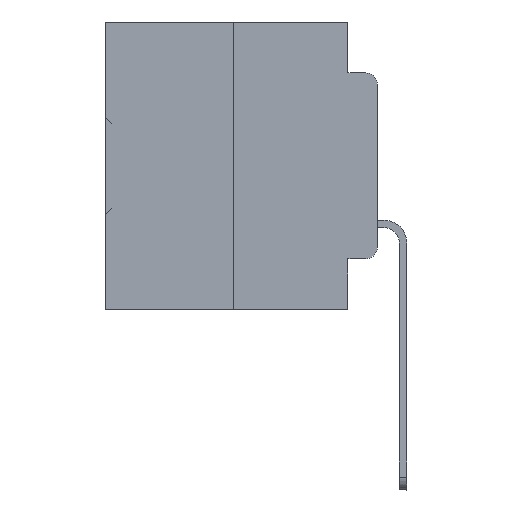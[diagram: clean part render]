
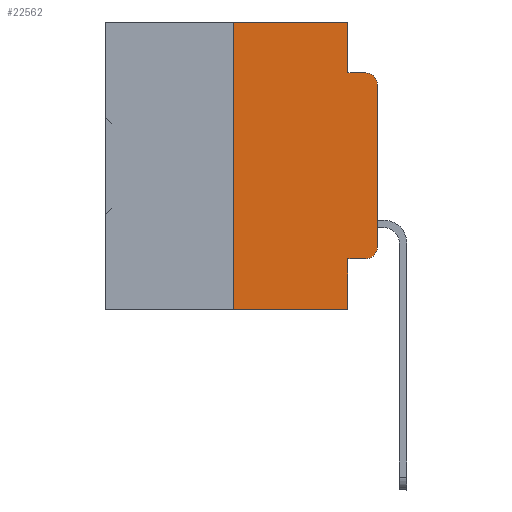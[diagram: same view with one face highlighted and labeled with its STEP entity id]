
A CAD part, left-side view. The second image highlights one B-rep face of the part: STEP entity #22562.
In plain terms, the highlighted planar face has unit normal (-1, 0, 0).
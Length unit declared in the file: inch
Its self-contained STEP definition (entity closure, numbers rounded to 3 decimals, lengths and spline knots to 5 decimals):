
#402 = CARTESIAN_POINT ( 'NONE',  ( 0., 0.473, 0. ) ) ;
#460 = EDGE_CURVE ( 'NONE', #38475, #35663, #22220, .T. ) ;
#1138 = LINE ( 'NONE', #13096, #17707 ) ;
#1702 = DIRECTION ( 'NONE',  ( 0., 0., 1. ) ) ;
#1963 = ORIENTED_EDGE ( 'NONE', *, *, #19429, .T. ) ;
#1972 = VERTEX_POINT ( 'NONE', #7918 ) ;
#2332 = CARTESIAN_POINT ( 'NONE',  ( 0., 0.02, -0.4115 ) ) ;
#2623 = AXIS2_PLACEMENT_3D ( 'NONE', #5279, #17221, #29190 ) ;
#2674 = EDGE_CURVE ( 'NONE', #1972, #4587, #21550, .T. ) ;
#2733 = CARTESIAN_POINT ( 'NONE',  ( 0., 0.051, 0. ) ) ;
#2928 = CARTESIAN_POINT ( 'NONE',  ( 0., 0.25, -0.5 ) ) ;
#3065 = VERTEX_POINT ( 'NONE', #2332 ) ;
#4380 = CARTESIAN_POINT ( 'NONE',  ( 0., 0.02, -0.1085 ) ) ;
#4405 = CARTESIAN_POINT ( 'NONE',  ( 0., 0.051, -0.0885 ) ) ;
#4587 = VERTEX_POINT ( 'NONE', #2733 ) ;
#5279 = CARTESIAN_POINT ( 'NONE',  ( 0., 0.473, 0. ) ) ;
#5509 = VECTOR ( 'NONE', #1702, 39.37008 ) ;
#7273 = DIRECTION ( 'NONE',  ( 0., 0., 1. ) ) ;
#7759 = CARTESIAN_POINT ( 'NONE',  ( 0., 0.051, 0. ) ) ;
#7784 = EDGE_CURVE ( 'NONE', #4587, #38475, #34631, .T. ) ;
#7918 = CARTESIAN_POINT ( 'NONE',  ( 0., 0.25, 0. ) ) ;
#9548 = ORIENTED_EDGE ( 'NONE', *, *, #28734, .T. ) ;
#11099 = CARTESIAN_POINT ( 'NONE',  ( 0., 0., -0.3915 ) ) ;
#11233 = ORIENTED_EDGE ( 'NONE', *, *, #2674, .F. ) ;
#11368 = FACE_OUTER_BOUND ( 'NONE', #25477, .T. ) ;
#11465 = CARTESIAN_POINT ( 'NONE',  ( 0., 0.02, -0.3915 ) ) ;
#11811 = VECTOR ( 'NONE', #32470, 39.37008 ) ;
#12011 = VERTEX_POINT ( 'NONE', #11099 ) ;
#12350 = ORIENTED_EDGE ( 'NONE', *, *, #460, .F. ) ;
#13096 = CARTESIAN_POINT ( 'NONE',  ( 0., 0.051, 0. ) ) ;
#14421 = CARTESIAN_POINT ( 'NONE',  ( 0., 0.051, -0.4115 ) ) ;
#14782 = LINE ( 'NONE', #20873, #11811 ) ;
#15048 = ORIENTED_EDGE ( 'NONE', *, *, #22030, .T. ) ;
#15068 = CARTESIAN_POINT ( 'NONE',  ( 0., 0., -0.1085 ) ) ;
#17221 = DIRECTION ( 'NONE',  ( 1., 0., 0. ) ) ;
#17608 = VECTOR ( 'NONE', #28331, 39.37008 ) ;
#17707 = VECTOR ( 'NONE', #25057, 39.37008 ) ;
#17903 = DIRECTION ( 'NONE',  ( 0., 0., -1. ) ) ;
#18599 = CARTESIAN_POINT ( 'NONE',  ( 0., 0.02, -0.0885 ) ) ;
#18655 = VECTOR ( 'NONE', #24978, 39.37008 ) ;
#18987 = ORIENTED_EDGE ( 'NONE', *, *, #37159, .F. ) ;
#19106 = LINE ( 'NONE', #30720, #17608 ) ;
#19393 = ORIENTED_EDGE ( 'NONE', *, *, #29683, .T. ) ;
#19429 = EDGE_CURVE ( 'NONE', #12011, #28964, #28443, .T. ) ;
#19528 = LINE ( 'NONE', #22272, #5509 ) ;
#19612 = CARTESIAN_POINT ( 'NONE',  ( 0., 0., 0. ) ) ;
#20181 = PLANE ( 'NONE',  #2623 ) ;
#20287 = DIRECTION ( 'NONE',  ( 0., 0., -1. ) ) ;
#20873 = CARTESIAN_POINT ( 'NONE',  ( 0., 0.473, -0.5 ) ) ;
#21100 = VERTEX_POINT ( 'NONE', #34524 ) ;
#21119 = ORIENTED_EDGE ( 'NONE', *, *, #7784, .F. ) ;
#21550 = LINE ( 'NONE', #402, #25412 ) ;
#22030 = EDGE_CURVE ( 'NONE', #38640, #3065, #19106, .T. ) ;
#22220 = LINE ( 'NONE', #4405, #18655 ) ;
#22272 = CARTESIAN_POINT ( 'NONE',  ( 0., 0.25, 0. ) ) ;
#22490 = CARTESIAN_POINT ( 'NONE',  ( 0., 0.051, -0.0885 ) ) ;
#22562 = ADVANCED_FACE ( 'NONE', ( #11368 ), #20181, .F. ) ;
#23126 = ORIENTED_EDGE ( 'NONE', *, *, #36206, .T. ) ;
#24978 = DIRECTION ( 'NONE',  ( 0., -1., 0. ) ) ;
#25057 = DIRECTION ( 'NONE',  ( 0., 0., -1. ) ) ;
#25412 = VECTOR ( 'NONE', #30796, 39.37008 ) ;
#25477 = EDGE_LOOP ( 'NONE', ( #1963, #9548, #12350, #21119, #11233, #18987, #23126, #29364, #15048, #19393 ) ) ;
#25954 = VECTOR ( 'NONE', #20287, 39.37008 ) ;
#28331 = DIRECTION ( 'NONE',  ( 0., -1., 0. ) ) ;
#28443 = LINE ( 'NONE', #19612, #28793 ) ;
#28734 = EDGE_CURVE ( 'NONE', #28964, #35663, #30046, .T. ) ;
#28793 = VECTOR ( 'NONE', #7273, 39.37008 ) ;
#28952 = VERTEX_POINT ( 'NONE', #2928 ) ;
#28964 = VERTEX_POINT ( 'NONE', #15068 ) ;
#29002 = DIRECTION ( 'NONE',  ( -1., 0., 0. ) ) ;
#29093 = EDGE_CURVE ( 'NONE', #38640, #21100, #1138, .T. ) ;
#29190 = DIRECTION ( 'NONE',  ( 0., 0., -1. ) ) ;
#29364 = ORIENTED_EDGE ( 'NONE', *, *, #29093, .F. ) ;
#29667 = AXIS2_PLACEMENT_3D ( 'NONE', #11465, #29686, #17903 ) ;
#29683 = EDGE_CURVE ( 'NONE', #3065, #12011, #34036, .T. ) ;
#29686 = DIRECTION ( 'NONE',  ( -1., 0., 0. ) ) ;
#30046 = CIRCLE ( 'NONE', #35054, 0.02 ) ;
#30720 = CARTESIAN_POINT ( 'NONE',  ( 0., 0.051, -0.4115 ) ) ;
#30796 = DIRECTION ( 'NONE',  ( 0., -1., 0. ) ) ;
#32470 = DIRECTION ( 'NONE',  ( 0., -1., 0. ) ) ;
#33983 = DIRECTION ( 'NONE',  ( 0., 0., -1. ) ) ;
#34036 = CIRCLE ( 'NONE', #29667, 0.02 ) ;
#34524 = CARTESIAN_POINT ( 'NONE',  ( 0., 0.051, -0.5 ) ) ;
#34631 = LINE ( 'NONE', #7759, #25954 ) ;
#35054 = AXIS2_PLACEMENT_3D ( 'NONE', #4380, #29002, #33983 ) ;
#35663 = VERTEX_POINT ( 'NONE', #18599 ) ;
#36206 = EDGE_CURVE ( 'NONE', #28952, #21100, #14782, .T. ) ;
#37159 = EDGE_CURVE ( 'NONE', #28952, #1972, #19528, .T. ) ;
#38475 = VERTEX_POINT ( 'NONE', #22490 ) ;
#38640 = VERTEX_POINT ( 'NONE', #14421 ) ;
